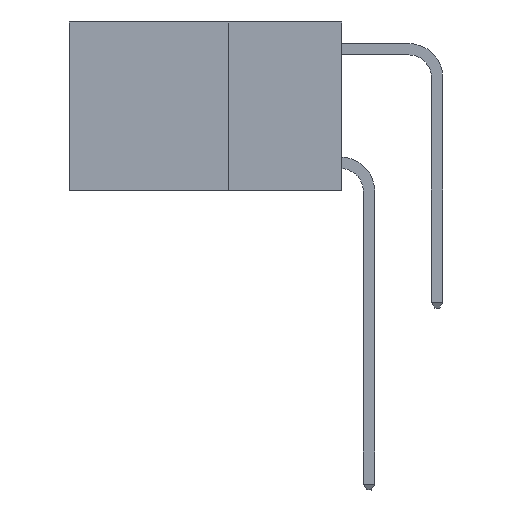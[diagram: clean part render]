
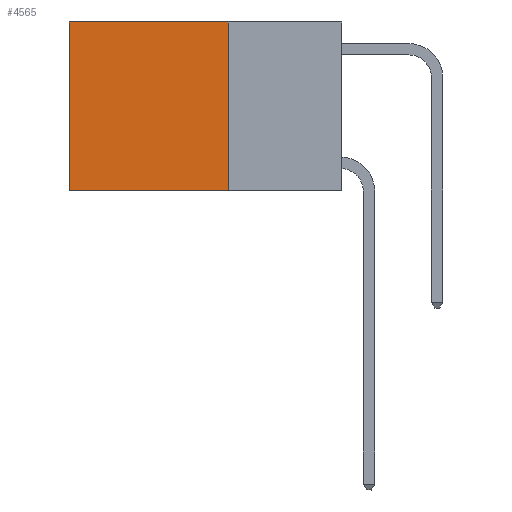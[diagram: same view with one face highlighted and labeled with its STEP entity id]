
A CAD part, left-side view. The second image highlights one B-rep face of the part: STEP entity #4565.
In plain terms, the highlighted planar face has unit normal (-1, 0, 0).
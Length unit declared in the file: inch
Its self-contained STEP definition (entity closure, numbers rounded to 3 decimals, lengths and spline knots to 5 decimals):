
#672 = DIRECTION ( 'NONE',  ( 0., 1., 0. ) ) ;
#1767 = EDGE_LOOP ( 'NONE', ( #21624, #22072, #16516, #24536 ) ) ;
#3919 = VERTEX_POINT ( 'NONE', #14878 ) ;
#4079 = VERTEX_POINT ( 'NONE', #25297 ) ;
#4565 = ADVANCED_FACE ( 'NONE', ( #11313 ), #4914, .F. ) ;
#4714 = DIRECTION ( 'NONE',  ( 0., 1., 0. ) ) ;
#4914 = PLANE ( 'NONE',  #19869 ) ;
#5599 = DIRECTION ( 'NONE',  ( 0., 0., -1. ) ) ;
#6404 = CARTESIAN_POINT ( 'NONE',  ( 0.2625, 0.25, 0. ) ) ;
#6778 = CARTESIAN_POINT ( 'NONE',  ( 0.2625, 0.6, 0. ) ) ;
#6940 = DIRECTION ( 'NONE',  ( 0., 0., -1. ) ) ;
#7958 = LINE ( 'NONE', #19805, #12754 ) ;
#8547 = DIRECTION ( 'NONE',  ( 0., 0., -1. ) ) ;
#11313 = FACE_OUTER_BOUND ( 'NONE', #1767, .T. ) ;
#12754 = VECTOR ( 'NONE', #5599, 39.37008 ) ;
#13873 = VECTOR ( 'NONE', #8547, 39.37008 ) ;
#14795 = EDGE_CURVE ( 'NONE', #18469, #3919, #19270, .T. ) ;
#14874 = LINE ( 'NONE', #24844, #24907 ) ;
#14878 = CARTESIAN_POINT ( 'NONE',  ( 0.2625, 0.25, -0.37 ) ) ;
#15504 = EDGE_CURVE ( 'NONE', #3919, #4079, #20182, .T. ) ;
#16516 = ORIENTED_EDGE ( 'NONE', *, *, #14795, .F. ) ;
#16862 = CARTESIAN_POINT ( 'NONE',  ( 0.2625, 0.25, -0.37 ) ) ;
#18241 = EDGE_CURVE ( 'NONE', #22043, #4079, #7958, .T. ) ;
#18469 = VERTEX_POINT ( 'NONE', #22559 ) ;
#19103 = DIRECTION ( 'NONE',  ( 1., 0., 0. ) ) ;
#19270 = LINE ( 'NONE', #6404, #13873 ) ;
#19561 = VECTOR ( 'NONE', #4714, 39.37008 ) ;
#19805 = CARTESIAN_POINT ( 'NONE',  ( 0.2625, 0.6, 0. ) ) ;
#19808 = EDGE_CURVE ( 'NONE', #18469, #22043, #14874, .T. ) ;
#19869 = AXIS2_PLACEMENT_3D ( 'NONE', #23038, #19103, #6940 ) ;
#20182 = LINE ( 'NONE', #16862, #19561 ) ;
#21624 = ORIENTED_EDGE ( 'NONE', *, *, #18241, .T. ) ;
#22043 = VERTEX_POINT ( 'NONE', #6778 ) ;
#22072 = ORIENTED_EDGE ( 'NONE', *, *, #15504, .F. ) ;
#22559 = CARTESIAN_POINT ( 'NONE',  ( 0.2625, 0.25, 0. ) ) ;
#23038 = CARTESIAN_POINT ( 'NONE',  ( 0.2625, 0.25, 0. ) ) ;
#24536 = ORIENTED_EDGE ( 'NONE', *, *, #19808, .T. ) ;
#24844 = CARTESIAN_POINT ( 'NONE',  ( 0.2625, 0.25, 0. ) ) ;
#24907 = VECTOR ( 'NONE', #672, 39.37008 ) ;
#25297 = CARTESIAN_POINT ( 'NONE',  ( 0.2625, 0.6, -0.37 ) ) ;
